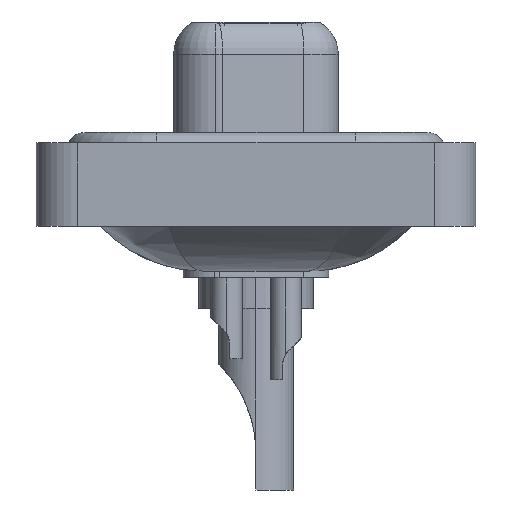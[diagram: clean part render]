
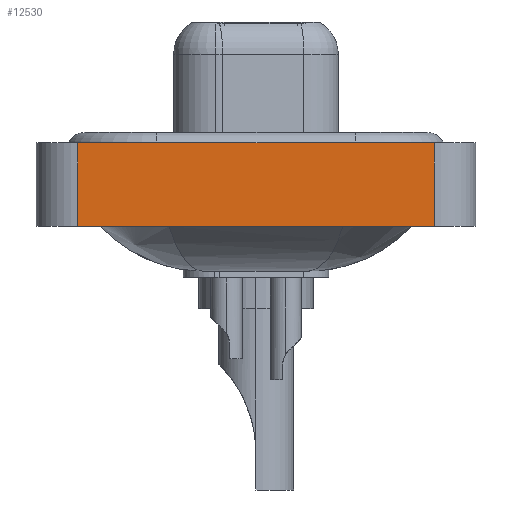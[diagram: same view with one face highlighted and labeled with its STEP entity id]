
A CAD part, left-side view. The second image highlights one B-rep face of the part: STEP entity #12530.
In plain terms, the highlighted planar face has unit normal (-1, 0, 0).
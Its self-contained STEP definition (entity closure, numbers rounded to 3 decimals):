
#154 = CARTESIAN_POINT ( 'NONE',  ( -7.3, -8.55, 0.4 ) ) ;
#892 = EDGE_CURVE ( 'NONE', #10168, #20144, #19831, .T. ) ;
#2259 = FACE_OUTER_BOUND ( 'NONE', #8788, .T. ) ;
#2478 = DIRECTION ( 'NONE',  ( -1., 0., 0. ) ) ;
#2900 = CARTESIAN_POINT ( 'NONE',  ( -7.3, 8.55, -3.6 ) ) ;
#3228 = VECTOR ( 'NONE', #8403, 1000. ) ;
#4248 = AXIS2_PLACEMENT_3D ( 'NONE', #14782, #2478, #11578 ) ;
#4291 = CARTESIAN_POINT ( 'NONE',  ( -7.3, -8.55, -3.6 ) ) ;
#4489 = CARTESIAN_POINT ( 'NONE',  ( -7.3, 8.55, -3.6 ) ) ;
#5453 = DIRECTION ( 'NONE',  ( 0., -1., 0. ) ) ;
#6430 = VECTOR ( 'NONE', #15207, 1000. ) ;
#8367 = CARTESIAN_POINT ( 'NONE',  ( -7.3, 8.55, 0.4 ) ) ;
#8403 = DIRECTION ( 'NONE',  ( 0., 0., 1. ) ) ;
#8788 = EDGE_LOOP ( 'NONE', ( #12790, #15105, #13321, #18043 ) ) ;
#9292 = PLANE ( 'NONE',  #4248 ) ;
#9825 = LINE ( 'NONE', #2900, #6430 ) ;
#10168 = VERTEX_POINT ( 'NONE', #4489 ) ;
#10245 = CARTESIAN_POINT ( 'NONE',  ( -7.3, -8.55, -3.6 ) ) ;
#10682 = VECTOR ( 'NONE', #11406, 1000. ) ;
#10800 = VERTEX_POINT ( 'NONE', #8367 ) ;
#11271 = EDGE_CURVE ( 'NONE', #10168, #10800, #9825, .T. ) ;
#11406 = DIRECTION ( 'NONE',  ( 0., -1., 0. ) ) ;
#11578 = DIRECTION ( 'NONE',  ( 0., 0., 1. ) ) ;
#12530 = ADVANCED_FACE ( 'NONE', ( #2259 ), #9292, .T. ) ;
#12790 = ORIENTED_EDGE ( 'NONE', *, *, #13809, .T. ) ;
#13321 = ORIENTED_EDGE ( 'NONE', *, *, #11271, .F. ) ;
#13809 = EDGE_CURVE ( 'NONE', #20144, #15692, #20955, .T. ) ;
#14621 = CARTESIAN_POINT ( 'NONE',  ( -7.3, -8.55, -3.6 ) ) ;
#14782 = CARTESIAN_POINT ( 'NONE',  ( -7.3, -8.55, -3.6 ) ) ;
#15105 = ORIENTED_EDGE ( 'NONE', *, *, #19955, .F. ) ;
#15207 = DIRECTION ( 'NONE',  ( 0., 0., 1. ) ) ;
#15692 = VERTEX_POINT ( 'NONE', #18875 ) ;
#17887 = LINE ( 'NONE', #154, #18467 ) ;
#18043 = ORIENTED_EDGE ( 'NONE', *, *, #892, .T. ) ;
#18467 = VECTOR ( 'NONE', #5453, 1000. ) ;
#18875 = CARTESIAN_POINT ( 'NONE',  ( -7.3, -8.55, 0.4 ) ) ;
#19831 = LINE ( 'NONE', #14621, #10682 ) ;
#19955 = EDGE_CURVE ( 'NONE', #10800, #15692, #17887, .T. ) ;
#20144 = VERTEX_POINT ( 'NONE', #4291 ) ;
#20955 = LINE ( 'NONE', #10245, #3228 ) ;
